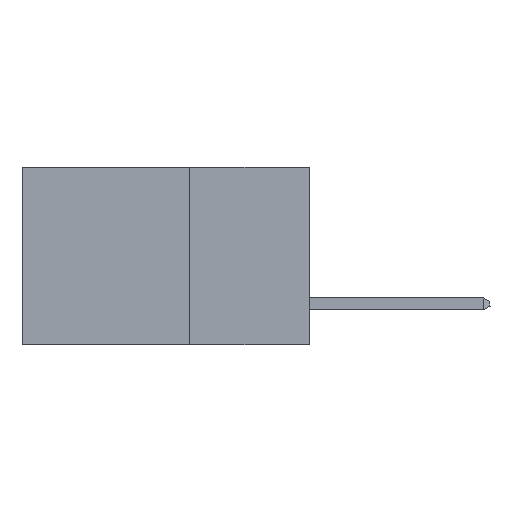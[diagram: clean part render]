
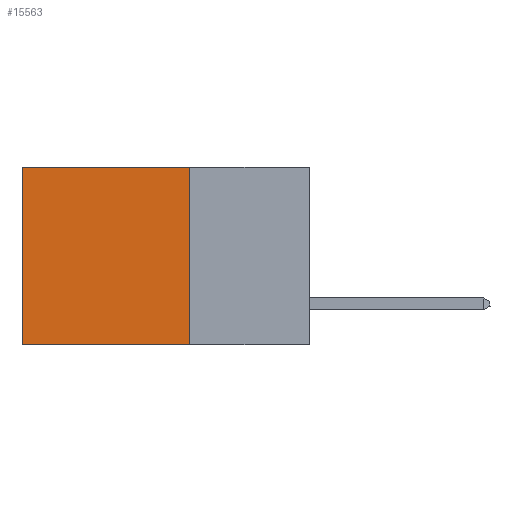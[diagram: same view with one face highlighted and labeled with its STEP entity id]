
A CAD part, left-side view. The second image highlights one B-rep face of the part: STEP entity #15563.
In plain terms, the highlighted planar face has unit normal (-1, 0, 0).
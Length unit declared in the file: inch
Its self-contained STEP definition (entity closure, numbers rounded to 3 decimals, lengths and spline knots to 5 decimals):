
#919 = VERTEX_POINT ( 'NONE', #20705 ) ;
#1048 = ORIENTED_EDGE ( 'NONE', *, *, #8982, .F. ) ;
#1704 = CARTESIAN_POINT ( 'NONE',  ( 0.2875, 0.6, 0. ) ) ;
#3271 = CARTESIAN_POINT ( 'NONE',  ( 0.2875, 0.25, 0. ) ) ;
#4088 = AXIS2_PLACEMENT_3D ( 'NONE', #30089, #32483, #14981 ) ;
#5416 = EDGE_CURVE ( 'NONE', #13256, #26458, #18800, .T. ) ;
#6734 = CARTESIAN_POINT ( 'NONE',  ( 0.2875, 0.25, -0.37 ) ) ;
#7515 = LINE ( 'NONE', #13017, #25674 ) ;
#8520 = DIRECTION ( 'NONE',  ( 0., 1., 0. ) ) ;
#8982 = EDGE_CURVE ( 'NONE', #919, #13256, #25650, .T. ) ;
#9512 = ORIENTED_EDGE ( 'NONE', *, *, #24670, .T. ) ;
#10575 = DIRECTION ( 'NONE',  ( 0., 0., -1. ) ) ;
#10727 = DIRECTION ( 'NONE',  ( 0., 1., 0. ) ) ;
#10826 = CARTESIAN_POINT ( 'NONE',  ( 0.2875, 0.25, -0.37 ) ) ;
#12318 = PLANE ( 'NONE',  #4088 ) ;
#12653 = VECTOR ( 'NONE', #18683, 39.37008 ) ;
#13017 = CARTESIAN_POINT ( 'NONE',  ( 0.2875, 0.6, 0. ) ) ;
#13256 = VERTEX_POINT ( 'NONE', #6734 ) ;
#14738 = CARTESIAN_POINT ( 'NONE',  ( 0.2875, 0.6, -0.37 ) ) ;
#14981 = DIRECTION ( 'NONE',  ( 0., 0., -1. ) ) ;
#15064 = VERTEX_POINT ( 'NONE', #1704 ) ;
#15563 = ADVANCED_FACE ( 'NONE', ( #32196 ), #12318, .F. ) ;
#16048 = VECTOR ( 'NONE', #10727, 39.37008 ) ;
#18683 = DIRECTION ( 'NONE',  ( 0., 0., -1. ) ) ;
#18800 = LINE ( 'NONE', #10826, #16048 ) ;
#18852 = ORIENTED_EDGE ( 'NONE', *, *, #5416, .F. ) ;
#18917 = CARTESIAN_POINT ( 'NONE',  ( 0.2875, 0.25, 0. ) ) ;
#20705 = CARTESIAN_POINT ( 'NONE',  ( 0.2875, 0.25, 0. ) ) ;
#23727 = LINE ( 'NONE', #3271, #29659 ) ;
#24131 = EDGE_CURVE ( 'NONE', #919, #15064, #23727, .T. ) ;
#24670 = EDGE_CURVE ( 'NONE', #15064, #26458, #7515, .T. ) ;
#25650 = LINE ( 'NONE', #18917, #12653 ) ;
#25674 = VECTOR ( 'NONE', #10575, 39.37008 ) ;
#26458 = VERTEX_POINT ( 'NONE', #14738 ) ;
#29659 = VECTOR ( 'NONE', #8520, 39.37008 ) ;
#29737 = EDGE_LOOP ( 'NONE', ( #9512, #18852, #1048, #32816 ) ) ;
#30089 = CARTESIAN_POINT ( 'NONE',  ( 0.2875, 0.25, 0. ) ) ;
#32196 = FACE_OUTER_BOUND ( 'NONE', #29737, .T. ) ;
#32483 = DIRECTION ( 'NONE',  ( 1., 0., 0. ) ) ;
#32816 = ORIENTED_EDGE ( 'NONE', *, *, #24131, .T. ) ;
